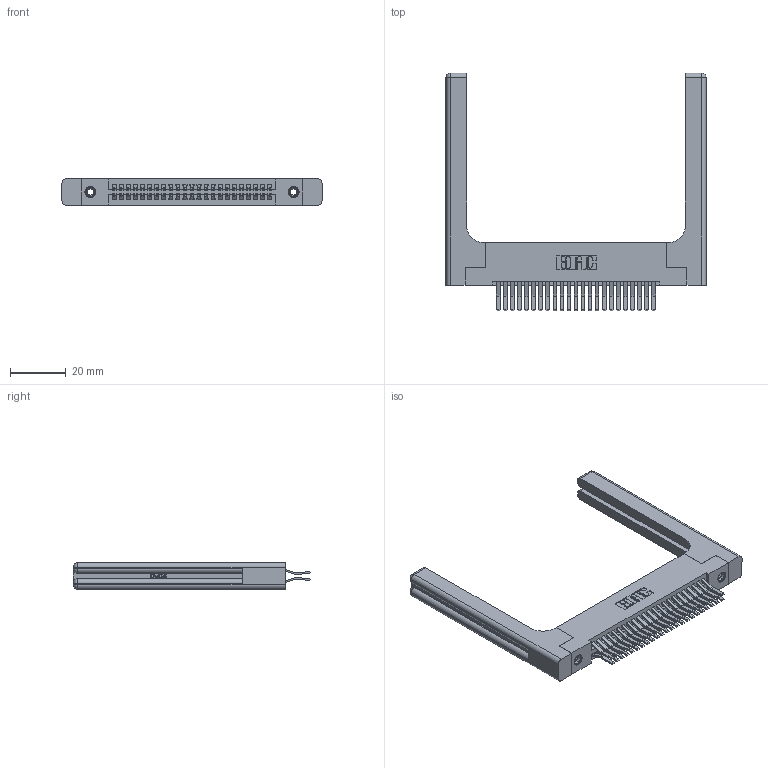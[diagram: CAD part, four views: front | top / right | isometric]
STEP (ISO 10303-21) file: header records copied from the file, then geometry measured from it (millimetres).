
FILE_DESCRIPTION (( 'STEP AP203' ), '1' );
FILE_NAME ('395-046-560-258.STEP', '2019-10-19T04:54:03', ( '' ), ( '' ), 'SwSTEP 2.0', 'SolidWorks 2016', '' );
FILE_SCHEMA (( 'CONFIG_CONTROL_DESIGN' ));
Length unit declared in the file: inch
Products named in the file (5): 345 Part_Flush Mounting Lugs - 0.156 Dia-TH; 345-292-001_560 Tail; 345-250-001_345-250-001-102; 345-220-058_345-220-058; 395-046-560-258
Assembly tree (51 placements, depth 2):
  395-046-560-258
    345 Part_Flush Mounting Lugs - 0.156 Dia-TH
    345-292-001_560 Tail  x46
    345-250-001_345-250-001-102  x2
    345-220-058_345-220-058  x2
Bounding box: 93.45 x 85.41 x 9.4 mm (x, y, z)
Volume: 17677.8 mm3; surface area: 19069.4 mm2
Topology: 51 solids, 51 shells, 2774 faces, 8137 edges, 5342 vertices
Faces by surface type: plane 1746, cylinder 968, bspline 36, cone 12, sphere 8, torus 4
Entity records: 25874 total; most frequent: CARTESIAN_POINT 5349, ORIENTED_EDGE 4080, DIRECTION 3676, EDGE_CURVE 2040, LINE 1720, VECTOR 1720, VERTEX_POINT 1350, AXIS2_PLACEMENT_3D 978
